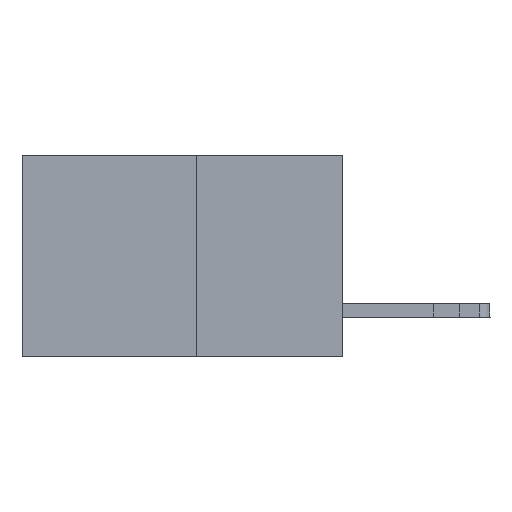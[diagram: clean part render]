
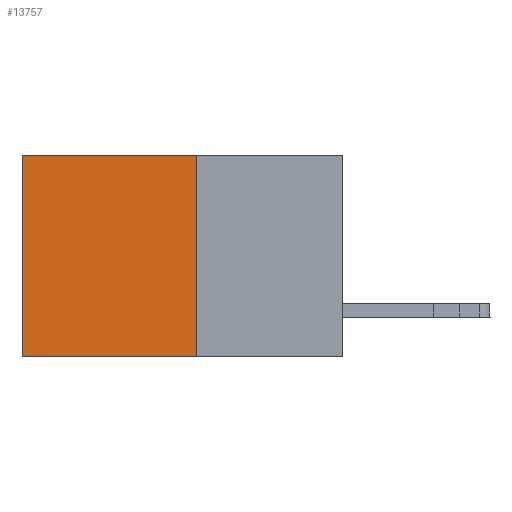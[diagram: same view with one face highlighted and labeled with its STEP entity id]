
A CAD part, left-side view. The second image highlights one B-rep face of the part: STEP entity #13757.
In plain terms, the highlighted planar face has unit normal (-1, 0, 0).
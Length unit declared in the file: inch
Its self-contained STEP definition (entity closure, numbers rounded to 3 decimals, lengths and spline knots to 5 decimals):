
#1092 = VECTOR ( 'NONE', #6301, 39.37008 ) ;
#1683 = VERTEX_POINT ( 'NONE', #4332 ) ;
#2403 = AXIS2_PLACEMENT_3D ( 'NONE', #15185, #20043, #18262 ) ;
#3787 = DIRECTION ( 'NONE',  ( 0., 0., -1. ) ) ;
#4332 = CARTESIAN_POINT ( 'NONE',  ( 0.277, 0.27, 0. ) ) ;
#4482 = CARTESIAN_POINT ( 'NONE',  ( 0.277, 0.27, -0.37 ) ) ;
#5566 = PLANE ( 'NONE',  #2403 ) ;
#6301 = DIRECTION ( 'NONE',  ( 0., 0., -1. ) ) ;
#7776 = ORIENTED_EDGE ( 'NONE', *, *, #12649, .T. ) ;
#7861 = CARTESIAN_POINT ( 'NONE',  ( 0.277, 0.59, 0. ) ) ;
#7872 = CARTESIAN_POINT ( 'NONE',  ( 0.277, 0.59, -0.37 ) ) ;
#7882 = CARTESIAN_POINT ( 'NONE',  ( 0.277, 0.27, -0.37 ) ) ;
#8599 = LINE ( 'NONE', #12305, #17888 ) ;
#9458 = LINE ( 'NONE', #7872, #1092 ) ;
#9677 = VERTEX_POINT ( 'NONE', #7882 ) ;
#9960 = EDGE_CURVE ( 'NONE', #1683, #18902, #8599, .T. ) ;
#11812 = LINE ( 'NONE', #18284, #19621 ) ;
#12305 = CARTESIAN_POINT ( 'NONE',  ( 0.277, 0.27, 0. ) ) ;
#12649 = EDGE_CURVE ( 'NONE', #18902, #17576, #9458, .T. ) ;
#12996 = EDGE_CURVE ( 'NONE', #9677, #17576, #15680, .T. ) ;
#13757 = ADVANCED_FACE ( 'NONE', ( #18367 ), #5566, .F. ) ;
#14126 = EDGE_CURVE ( 'NONE', #1683, #9677, #11812, .T. ) ;
#14708 = CARTESIAN_POINT ( 'NONE',  ( 0.277, 0.59, -0.37 ) ) ;
#14925 = VECTOR ( 'NONE', #20544, 39.37008 ) ;
#15185 = CARTESIAN_POINT ( 'NONE',  ( 0.277, 0.27, -0.37 ) ) ;
#15238 = ORIENTED_EDGE ( 'NONE', *, *, #14126, .F. ) ;
#15374 = DIRECTION ( 'NONE',  ( 0., 1., 0. ) ) ;
#15680 = LINE ( 'NONE', #4482, #14925 ) ;
#15737 = ORIENTED_EDGE ( 'NONE', *, *, #12996, .F. ) ;
#17576 = VERTEX_POINT ( 'NONE', #14708 ) ;
#17888 = VECTOR ( 'NONE', #15374, 39.37008 ) ;
#18124 = EDGE_LOOP ( 'NONE', ( #7776, #15737, #15238, #20474 ) ) ;
#18262 = DIRECTION ( 'NONE',  ( 0., 0., -1. ) ) ;
#18284 = CARTESIAN_POINT ( 'NONE',  ( 0.277, 0.27, -0.37 ) ) ;
#18367 = FACE_OUTER_BOUND ( 'NONE', #18124, .T. ) ;
#18902 = VERTEX_POINT ( 'NONE', #7861 ) ;
#19621 = VECTOR ( 'NONE', #3787, 39.37008 ) ;
#20043 = DIRECTION ( 'NONE',  ( 1., 0., 0. ) ) ;
#20474 = ORIENTED_EDGE ( 'NONE', *, *, #9960, .T. ) ;
#20544 = DIRECTION ( 'NONE',  ( 0., 1., 0. ) ) ;
